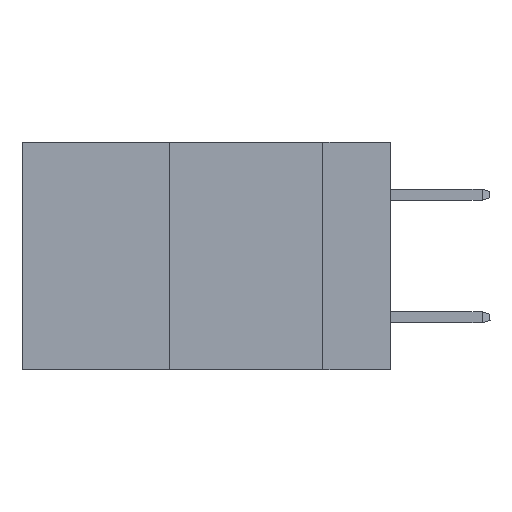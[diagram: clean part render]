
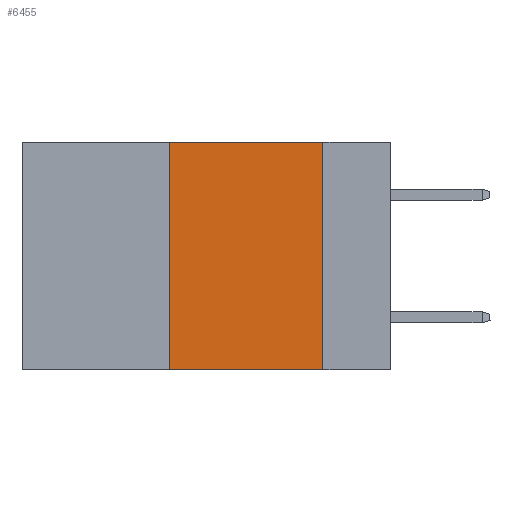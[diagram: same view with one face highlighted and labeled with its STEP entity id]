
A CAD part, left-side view. The second image highlights one B-rep face of the part: STEP entity #6455.
In plain terms, the highlighted planar face has unit normal (-1, 0, 0).
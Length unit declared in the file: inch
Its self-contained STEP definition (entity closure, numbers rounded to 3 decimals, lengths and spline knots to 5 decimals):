
#11 = VERTEX_POINT ( 'NONE', #2255 ) ;
#256 = ORIENTED_EDGE ( 'NONE', *, *, #2591, .F. ) ;
#327 = ORIENTED_EDGE ( 'NONE', *, *, #1504, .F. ) ;
#672 = DIRECTION ( 'NONE',  ( 0., -1., 0. ) ) ;
#1069 = LINE ( 'NONE', #8993, #8175 ) ;
#1183 = VERTEX_POINT ( 'NONE', #6624 ) ;
#1373 = ORIENTED_EDGE ( 'NONE', *, *, #4628, .T. ) ;
#1504 = EDGE_CURVE ( 'NONE', #4717, #1951, #8574, .T. ) ;
#1951 = VERTEX_POINT ( 'NONE', #3729 ) ;
#2219 = CARTESIAN_POINT ( 'NONE',  ( 0., 0.36, 0. ) ) ;
#2255 = CARTESIAN_POINT ( 'NONE',  ( 0., 0.11, -0.37 ) ) ;
#2459 = DIRECTION ( 'NONE',  ( 0., 0., -1. ) ) ;
#2591 = EDGE_CURVE ( 'NONE', #1183, #4717, #7029, .T. ) ;
#3009 = DIRECTION ( 'NONE',  ( 0., 0., -1. ) ) ;
#3020 = DIRECTION ( 'NONE',  ( 1., 0., 0. ) ) ;
#3046 = CARTESIAN_POINT ( 'NONE',  ( 0., 0.11, 0. ) ) ;
#3100 = VECTOR ( 'NONE', #4141, 39.37008 ) ;
#3126 = EDGE_CURVE ( 'NONE', #1951, #11, #8189, .T. ) ;
#3235 = PLANE ( 'NONE',  #5731 ) ;
#3335 = CARTESIAN_POINT ( 'NONE',  ( 0., 0.6, 0. ) ) ;
#3729 = CARTESIAN_POINT ( 'NONE',  ( 0., 0.11, 0. ) ) ;
#3833 = CARTESIAN_POINT ( 'NONE',  ( 0., 0.6, 0. ) ) ;
#4141 = DIRECTION ( 'NONE',  ( 0., -1., 0. ) ) ;
#4628 = EDGE_CURVE ( 'NONE', #1183, #11, #1069, .T. ) ;
#4637 = VECTOR ( 'NONE', #3009, 39.37008 ) ;
#4717 = VERTEX_POINT ( 'NONE', #2219 ) ;
#5088 = ORIENTED_EDGE ( 'NONE', *, *, #3126, .F. ) ;
#5363 = EDGE_LOOP ( 'NONE', ( #5088, #327, #256, #1373 ) ) ;
#5731 = AXIS2_PLACEMENT_3D ( 'NONE', #3833, #3020, #2459 ) ;
#6455 = ADVANCED_FACE ( 'NONE', ( #9101 ), #3235, .F. ) ;
#6624 = CARTESIAN_POINT ( 'NONE',  ( 0., 0.36, -0.37 ) ) ;
#6813 = VECTOR ( 'NONE', #8836, 39.37008 ) ;
#6967 = CARTESIAN_POINT ( 'NONE',  ( 0., 0.36, 0. ) ) ;
#7029 = LINE ( 'NONE', #6967, #6813 ) ;
#8175 = VECTOR ( 'NONE', #672, 39.37008 ) ;
#8189 = LINE ( 'NONE', #3046, #4637 ) ;
#8574 = LINE ( 'NONE', #3335, #3100 ) ;
#8836 = DIRECTION ( 'NONE',  ( 0., 0., 1. ) ) ;
#8993 = CARTESIAN_POINT ( 'NONE',  ( 0., 0.6, -0.37 ) ) ;
#9101 = FACE_OUTER_BOUND ( 'NONE', #5363, .T. ) ;
